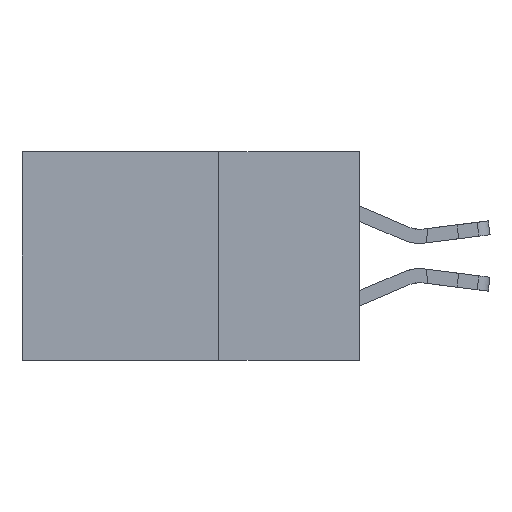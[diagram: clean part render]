
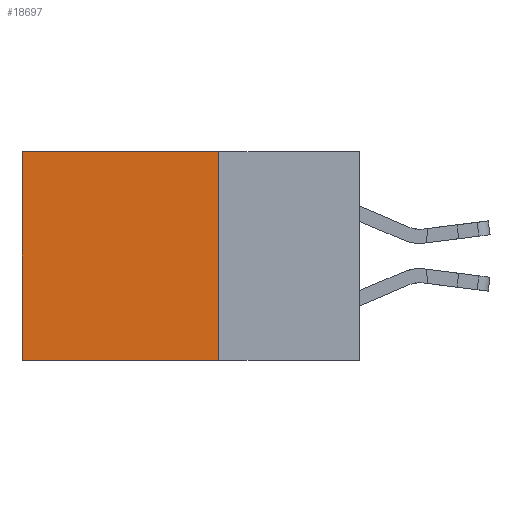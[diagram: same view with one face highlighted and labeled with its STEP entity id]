
A CAD part, left-side view. The second image highlights one B-rep face of the part: STEP entity #18697.
In plain terms, the highlighted planar face has unit normal (-1, 0, 0).
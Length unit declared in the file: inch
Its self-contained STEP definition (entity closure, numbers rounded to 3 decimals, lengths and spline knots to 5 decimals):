
#242 = DIRECTION ( 'NONE',  ( 0., 1., 0. ) ) ;
#1062 = DIRECTION ( 'NONE',  ( 0., 0., -1. ) ) ;
#1740 = LINE ( 'NONE', #6486, #23080 ) ;
#2192 = CARTESIAN_POINT ( 'NONE',  ( 0.2875, 0.25, 0. ) ) ;
#2715 = LINE ( 'NONE', #18547, #22389 ) ;
#3129 = PLANE ( 'NONE',  #20949 ) ;
#3650 = CARTESIAN_POINT ( 'NONE',  ( 0.2875, 0.25, 0. ) ) ;
#3986 = VERTEX_POINT ( 'NONE', #9281 ) ;
#4858 = ORIENTED_EDGE ( 'NONE', *, *, #11895, .T. ) ;
#5151 = CARTESIAN_POINT ( 'NONE',  ( 0.2875, 0.6, 0. ) ) ;
#5323 = LINE ( 'NONE', #3650, #7303 ) ;
#5457 = VERTEX_POINT ( 'NONE', #5151 ) ;
#6127 = ORIENTED_EDGE ( 'NONE', *, *, #9334, .F. ) ;
#6486 = CARTESIAN_POINT ( 'NONE',  ( 0.2875, 0.6, 0. ) ) ;
#7303 = VECTOR ( 'NONE', #11959, 39.37008 ) ;
#8171 = CARTESIAN_POINT ( 'NONE',  ( 0.2875, 0.25, 0. ) ) ;
#8264 = DIRECTION ( 'NONE',  ( 0., 1., 0. ) ) ;
#8591 = EDGE_CURVE ( 'NONE', #18144, #3986, #5323, .T. ) ;
#9281 = CARTESIAN_POINT ( 'NONE',  ( 0.2875, 0.25, -0.37 ) ) ;
#9334 = EDGE_CURVE ( 'NONE', #3986, #24511, #2715, .T. ) ;
#9640 = ORIENTED_EDGE ( 'NONE', *, *, #12627, .T. ) ;
#9726 = EDGE_LOOP ( 'NONE', ( #9640, #6127, #10159, #4858 ) ) ;
#10159 = ORIENTED_EDGE ( 'NONE', *, *, #8591, .F. ) ;
#11452 = DIRECTION ( 'NONE',  ( 1., 0., 0. ) ) ;
#11895 = EDGE_CURVE ( 'NONE', #18144, #5457, #14402, .T. ) ;
#11959 = DIRECTION ( 'NONE',  ( 0., 0., -1. ) ) ;
#12627 = EDGE_CURVE ( 'NONE', #5457, #24511, #1740, .T. ) ;
#14402 = LINE ( 'NONE', #8171, #16653 ) ;
#16653 = VECTOR ( 'NONE', #8264, 39.37008 ) ;
#17100 = CARTESIAN_POINT ( 'NONE',  ( 0.2875, 0.6, -0.37 ) ) ;
#18144 = VERTEX_POINT ( 'NONE', #2192 ) ;
#18547 = CARTESIAN_POINT ( 'NONE',  ( 0.2875, 0.25, -0.37 ) ) ;
#18697 = ADVANCED_FACE ( 'NONE', ( #22854 ), #3129, .F. ) ;
#20949 = AXIS2_PLACEMENT_3D ( 'NONE', #25776, #11452, #1062 ) ;
#21734 = DIRECTION ( 'NONE',  ( 0., 0., -1. ) ) ;
#22389 = VECTOR ( 'NONE', #242, 39.37008 ) ;
#22854 = FACE_OUTER_BOUND ( 'NONE', #9726, .T. ) ;
#23080 = VECTOR ( 'NONE', #21734, 39.37008 ) ;
#24511 = VERTEX_POINT ( 'NONE', #17100 ) ;
#25776 = CARTESIAN_POINT ( 'NONE',  ( 0.2875, 0.25, 0. ) ) ;
